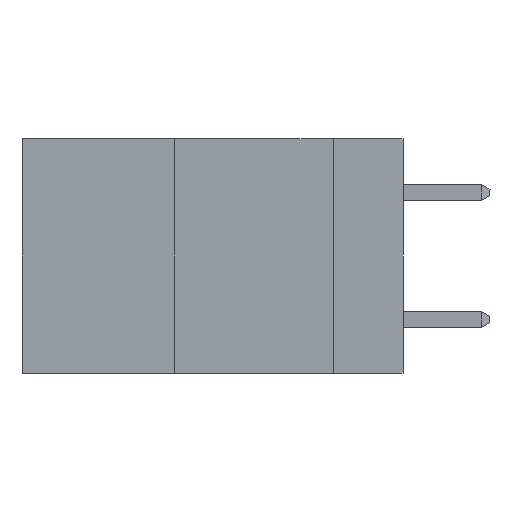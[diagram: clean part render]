
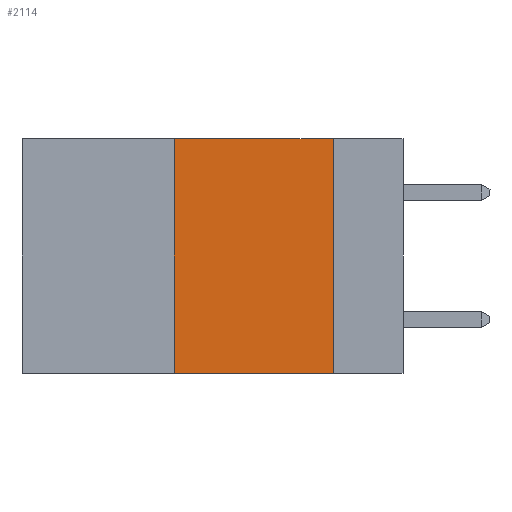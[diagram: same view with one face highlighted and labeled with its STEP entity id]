
A CAD part, left-side view. The second image highlights one B-rep face of the part: STEP entity #2114.
In plain terms, the highlighted planar face has unit normal (-1, 0, 0).
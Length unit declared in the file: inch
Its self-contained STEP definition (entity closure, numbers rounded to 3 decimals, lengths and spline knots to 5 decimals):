
#100 = EDGE_LOOP ( 'NONE', ( #2185, #1415, #11974, #11186 ) ) ;
#571 = VERTEX_POINT ( 'NONE', #8652 ) ;
#707 = DIRECTION ( 'NONE',  ( 0., -1., 0. ) ) ;
#715 = DIRECTION ( 'NONE',  ( 0., 0., -1. ) ) ;
#1415 = ORIENTED_EDGE ( 'NONE', *, *, #9584, .F. ) ;
#1779 = VECTOR ( 'NONE', #8850, 39.37008 ) ;
#2114 = ADVANCED_FACE ( 'NONE', ( #8350 ), #4599, .F. ) ;
#2185 = ORIENTED_EDGE ( 'NONE', *, *, #9417, .F. ) ;
#2373 = VERTEX_POINT ( 'NONE', #6722 ) ;
#2521 = CARTESIAN_POINT ( 'NONE',  ( 0., 0.36, 0. ) ) ;
#2532 = VECTOR ( 'NONE', #707, 39.37008 ) ;
#2578 = LINE ( 'NONE', #2521, #6650 ) ;
#2655 = CARTESIAN_POINT ( 'NONE',  ( 0., 0.6, -0.37 ) ) ;
#3159 = CARTESIAN_POINT ( 'NONE',  ( 0., 0.6, 0. ) ) ;
#3394 = AXIS2_PLACEMENT_3D ( 'NONE', #4768, #3626, #715 ) ;
#3431 = EDGE_CURVE ( 'NONE', #571, #11943, #2578, .T. ) ;
#3529 = DIRECTION ( 'NONE',  ( 0., 0., 1. ) ) ;
#3626 = DIRECTION ( 'NONE',  ( 1., 0., 0. ) ) ;
#4122 = LINE ( 'NONE', #11922, #1779 ) ;
#4599 = PLANE ( 'NONE',  #3394 ) ;
#4768 = CARTESIAN_POINT ( 'NONE',  ( 0., 0.6, 0. ) ) ;
#4835 = EDGE_CURVE ( 'NONE', #571, #11886, #8162, .T. ) ;
#6650 = VECTOR ( 'NONE', #3529, 39.37008 ) ;
#6722 = CARTESIAN_POINT ( 'NONE',  ( 0., 0.11, 0. ) ) ;
#7066 = DIRECTION ( 'NONE',  ( 0., -1., 0. ) ) ;
#7110 = LINE ( 'NONE', #3159, #12503 ) ;
#7553 = CARTESIAN_POINT ( 'NONE',  ( 0., 0.36, 0. ) ) ;
#8162 = LINE ( 'NONE', #2655, #2532 ) ;
#8350 = FACE_OUTER_BOUND ( 'NONE', #100, .T. ) ;
#8652 = CARTESIAN_POINT ( 'NONE',  ( 0., 0.36, -0.37 ) ) ;
#8850 = DIRECTION ( 'NONE',  ( 0., 0., -1. ) ) ;
#9417 = EDGE_CURVE ( 'NONE', #2373, #11886, #4122, .T. ) ;
#9510 = CARTESIAN_POINT ( 'NONE',  ( 0., 0.11, -0.37 ) ) ;
#9584 = EDGE_CURVE ( 'NONE', #11943, #2373, #7110, .T. ) ;
#11186 = ORIENTED_EDGE ( 'NONE', *, *, #4835, .T. ) ;
#11886 = VERTEX_POINT ( 'NONE', #9510 ) ;
#11922 = CARTESIAN_POINT ( 'NONE',  ( 0., 0.11, 0. ) ) ;
#11943 = VERTEX_POINT ( 'NONE', #7553 ) ;
#11974 = ORIENTED_EDGE ( 'NONE', *, *, #3431, .F. ) ;
#12503 = VECTOR ( 'NONE', #7066, 39.37008 ) ;
